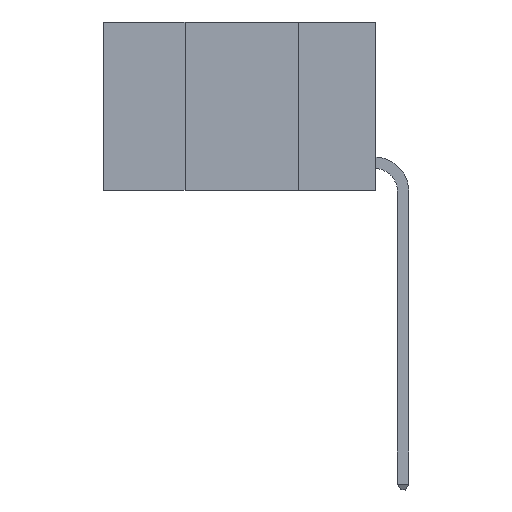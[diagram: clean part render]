
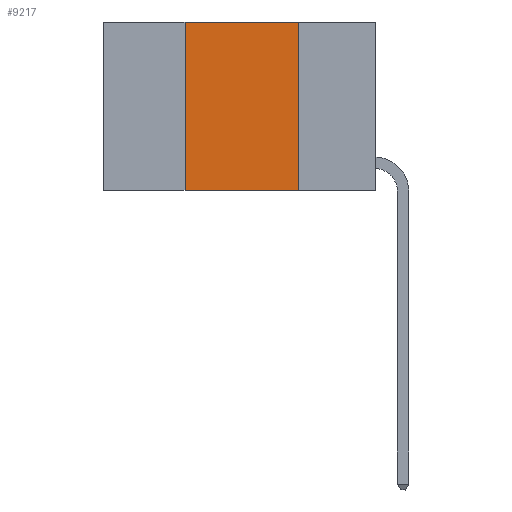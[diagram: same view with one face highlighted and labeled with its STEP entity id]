
A CAD part, left-side view. The second image highlights one B-rep face of the part: STEP entity #9217.
In plain terms, the highlighted planar face has unit normal (-1, 0, 0).
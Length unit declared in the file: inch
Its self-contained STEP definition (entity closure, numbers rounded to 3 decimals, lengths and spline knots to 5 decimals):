
#325 = EDGE_LOOP ( 'NONE', ( #12779, #7509, #10417, #4991 ) ) ;
#594 = DIRECTION ( 'NONE',  ( 0., -1., 0. ) ) ;
#748 = DIRECTION ( 'NONE',  ( 1., 0., 0. ) ) ;
#943 = FACE_OUTER_BOUND ( 'NONE', #325, .T. ) ;
#1786 = VECTOR ( 'NONE', #9105, 39.37008 ) ;
#2134 = VECTOR ( 'NONE', #3734, 39.37008 ) ;
#3041 = CARTESIAN_POINT ( 'NONE',  ( 0., 0.42, 0. ) ) ;
#3686 = VECTOR ( 'NONE', #3803, 39.37008 ) ;
#3734 = DIRECTION ( 'NONE',  ( 0., -1., 0. ) ) ;
#3803 = DIRECTION ( 'NONE',  ( 0., 0., -1. ) ) ;
#4119 = EDGE_CURVE ( 'NONE', #10537, #5809, #12183, .T. ) ;
#4991 = ORIENTED_EDGE ( 'NONE', *, *, #10889, .T. ) ;
#5003 = VERTEX_POINT ( 'NONE', #6062 ) ;
#5019 = LINE ( 'NONE', #5853, #2134 ) ;
#5248 = CARTESIAN_POINT ( 'NONE',  ( 0., 0.17, 0. ) ) ;
#5809 = VERTEX_POINT ( 'NONE', #9644 ) ;
#5853 = CARTESIAN_POINT ( 'NONE',  ( 0., 0.6, 0. ) ) ;
#6062 = CARTESIAN_POINT ( 'NONE',  ( 0., 0.42, -0.37 ) ) ;
#7310 = CARTESIAN_POINT ( 'NONE',  ( 0., 0.6, 0. ) ) ;
#7509 = ORIENTED_EDGE ( 'NONE', *, *, #12113, .F. ) ;
#8408 = DIRECTION ( 'NONE',  ( 0., 0., -1. ) ) ;
#8417 = VECTOR ( 'NONE', #594, 39.37008 ) ;
#8728 = VERTEX_POINT ( 'NONE', #3041 ) ;
#9105 = DIRECTION ( 'NONE',  ( 0., 0., 1. ) ) ;
#9217 = ADVANCED_FACE ( 'NONE', ( #943 ), #11552, .F. ) ;
#9644 = CARTESIAN_POINT ( 'NONE',  ( 0., 0.17, -0.37 ) ) ;
#10215 = CARTESIAN_POINT ( 'NONE',  ( 0., 0.42, 0. ) ) ;
#10306 = CARTESIAN_POINT ( 'NONE',  ( 0., 0.17, 0. ) ) ;
#10417 = ORIENTED_EDGE ( 'NONE', *, *, #12923, .F. ) ;
#10537 = VERTEX_POINT ( 'NONE', #5248 ) ;
#10889 = EDGE_CURVE ( 'NONE', #5003, #5809, #11252, .T. ) ;
#11252 = LINE ( 'NONE', #12399, #8417 ) ;
#11552 = PLANE ( 'NONE',  #11634 ) ;
#11634 = AXIS2_PLACEMENT_3D ( 'NONE', #7310, #748, #8408 ) ;
#12113 = EDGE_CURVE ( 'NONE', #8728, #10537, #5019, .T. ) ;
#12183 = LINE ( 'NONE', #10306, #3686 ) ;
#12399 = CARTESIAN_POINT ( 'NONE',  ( 0., 0.6, -0.37 ) ) ;
#12779 = ORIENTED_EDGE ( 'NONE', *, *, #4119, .F. ) ;
#12923 = EDGE_CURVE ( 'NONE', #5003, #8728, #13124, .T. ) ;
#13124 = LINE ( 'NONE', #10215, #1786 ) ;
